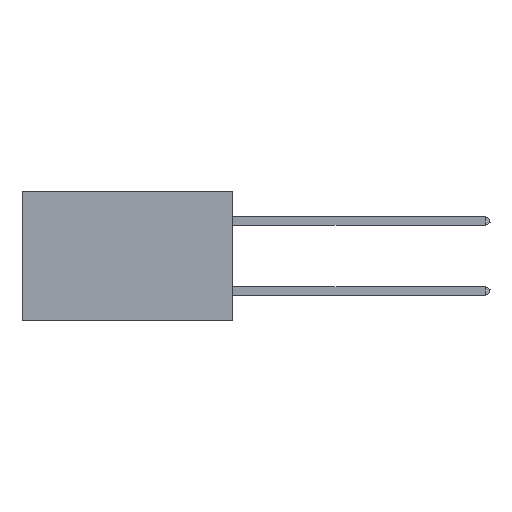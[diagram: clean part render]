
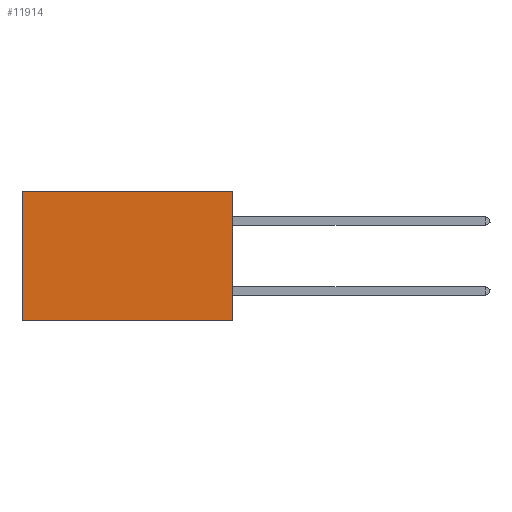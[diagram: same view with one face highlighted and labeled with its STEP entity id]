
A CAD part, left-side view. The second image highlights one B-rep face of the part: STEP entity #11914.
In plain terms, the highlighted planar face has unit normal (-1, 0, 0).
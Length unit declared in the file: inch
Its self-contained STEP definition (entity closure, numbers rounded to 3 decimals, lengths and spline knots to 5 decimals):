
#1133 = EDGE_LOOP ( 'NONE', ( #5301, #8972, #1991, #13596 ) ) ;
#1683 = CARTESIAN_POINT ( 'NONE',  ( 0.2875, 0., 0. ) ) ;
#1991 = ORIENTED_EDGE ( 'NONE', *, *, #9044, .F. ) ;
#2267 = DIRECTION ( 'NONE',  ( 0., 1., 0. ) ) ;
#2395 = CARTESIAN_POINT ( 'NONE',  ( 0.2875, 0.6, 0. ) ) ;
#2551 = DIRECTION ( 'NONE',  ( 0., 0., -1. ) ) ;
#2685 = CARTESIAN_POINT ( 'NONE',  ( 0.2875, 0., 0. ) ) ;
#3523 = VECTOR ( 'NONE', #2551, 39.37008 ) ;
#3597 = DIRECTION ( 'NONE',  ( 0., 0., -1. ) ) ;
#3640 = EDGE_CURVE ( 'NONE', #8531, #12497, #12882, .T. ) ;
#5301 = ORIENTED_EDGE ( 'NONE', *, *, #3640, .T. ) ;
#6014 = VECTOR ( 'NONE', #9306, 39.37008 ) ;
#6113 = VECTOR ( 'NONE', #14163, 39.37008 ) ;
#6616 = VECTOR ( 'NONE', #2267, 39.37008 ) ;
#6671 = VERTEX_POINT ( 'NONE', #11764 ) ;
#7117 = PLANE ( 'NONE',  #13506 ) ;
#7188 = EDGE_CURVE ( 'NONE', #6671, #12497, #9532, .T. ) ;
#7336 = CARTESIAN_POINT ( 'NONE',  ( 0.2875, 0.6, 0. ) ) ;
#8045 = VERTEX_POINT ( 'NONE', #2685 ) ;
#8531 = VERTEX_POINT ( 'NONE', #7336 ) ;
#8958 = LINE ( 'NONE', #12574, #6014 ) ;
#8972 = ORIENTED_EDGE ( 'NONE', *, *, #7188, .F. ) ;
#9044 = EDGE_CURVE ( 'NONE', #8045, #6671, #8958, .T. ) ;
#9302 = CARTESIAN_POINT ( 'NONE',  ( 0.2875, 0., 0. ) ) ;
#9306 = DIRECTION ( 'NONE',  ( 0., 0., -1. ) ) ;
#9532 = LINE ( 'NONE', #14689, #6616 ) ;
#10396 = DIRECTION ( 'NONE',  ( 1., 0., 0. ) ) ;
#10430 = EDGE_CURVE ( 'NONE', #8045, #8531, #14494, .T. ) ;
#11764 = CARTESIAN_POINT ( 'NONE',  ( 0.2875, 0., -0.37 ) ) ;
#11914 = ADVANCED_FACE ( 'NONE', ( #12089 ), #7117, .F. ) ;
#12089 = FACE_OUTER_BOUND ( 'NONE', #1133, .T. ) ;
#12497 = VERTEX_POINT ( 'NONE', #14061 ) ;
#12574 = CARTESIAN_POINT ( 'NONE',  ( 0.2875, 0., 0. ) ) ;
#12882 = LINE ( 'NONE', #2395, #3523 ) ;
#13506 = AXIS2_PLACEMENT_3D ( 'NONE', #9302, #10396, #3597 ) ;
#13596 = ORIENTED_EDGE ( 'NONE', *, *, #10430, .T. ) ;
#14061 = CARTESIAN_POINT ( 'NONE',  ( 0.2875, 0.6, -0.37 ) ) ;
#14163 = DIRECTION ( 'NONE',  ( 0., 1., 0. ) ) ;
#14494 = LINE ( 'NONE', #1683, #6113 ) ;
#14689 = CARTESIAN_POINT ( 'NONE',  ( 0.2875, 0., -0.37 ) ) ;
